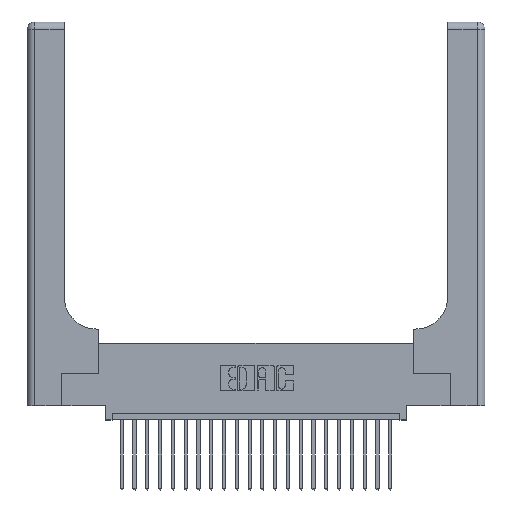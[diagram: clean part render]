
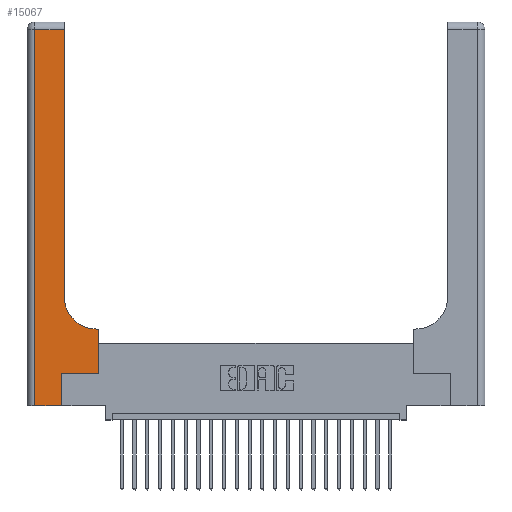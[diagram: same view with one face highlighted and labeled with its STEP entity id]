
A CAD part, top view. The second image highlights one B-rep face of the part: STEP entity #15067.
In plain terms, the highlighted planar face has unit normal (0, 0, 1).
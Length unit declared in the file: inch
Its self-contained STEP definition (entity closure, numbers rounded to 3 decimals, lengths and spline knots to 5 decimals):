
#415 = VECTOR ( 'NONE', #22402, 39.37008 ) ;
#859 = VECTOR ( 'NONE', #13262, 39.37008 ) ;
#1002 = LINE ( 'NONE', #6047, #415 ) ;
#1111 = PLANE ( 'NONE',  #16423 ) ;
#1129 = EDGE_CURVE ( 'NONE', #18419, #1137, #2459, .T. ) ;
#1137 = VERTEX_POINT ( 'NONE', #24298 ) ;
#1492 = CARTESIAN_POINT ( 'NONE',  ( 0., 0., 0.37 ) ) ;
#1927 = LINE ( 'NONE', #15598, #10284 ) ;
#2187 = CARTESIAN_POINT ( 'NONE',  ( 0.2915, 2.94, 0.37 ) ) ;
#2373 = ORIENTED_EDGE ( 'NONE', *, *, #10938, .T. ) ;
#2414 = CARTESIAN_POINT ( 'NONE',  ( 0.269, 0.25, 0.37 ) ) ;
#2459 = LINE ( 'NONE', #11232, #8430 ) ;
#2984 = DIRECTION ( 'NONE',  ( 1., 0., 0. ) ) ;
#3992 = CARTESIAN_POINT ( 'NONE',  ( 0.5415, 0.85, 0.37 ) ) ;
#4727 = CARTESIAN_POINT ( 'NONE',  ( 0.5585, 0.25, 0.37 ) ) ;
#5417 = VECTOR ( 'NONE', #24611, 39.37008 ) ;
#5508 = ORIENTED_EDGE ( 'NONE', *, *, #21727, .T. ) ;
#5813 = VERTEX_POINT ( 'NONE', #2414 ) ;
#6047 = CARTESIAN_POINT ( 'NONE',  ( 0.269, 0., 0.37 ) ) ;
#6265 = ORIENTED_EDGE ( 'NONE', *, *, #1129, .T. ) ;
#6415 = VECTOR ( 'NONE', #13257, 39.37008 ) ;
#6490 = ORIENTED_EDGE ( 'NONE', *, *, #20495, .T. ) ;
#6573 = VERTEX_POINT ( 'NONE', #10882 ) ;
#7051 = CARTESIAN_POINT ( 'NONE',  ( 0.06, 2.94, 0.37 ) ) ;
#7939 = VERTEX_POINT ( 'NONE', #13081 ) ;
#8109 = DIRECTION ( 'NONE',  ( -1., 0., 0. ) ) ;
#8239 = VECTOR ( 'NONE', #8879, 39.37008 ) ;
#8430 = VECTOR ( 'NONE', #18910, 39.37008 ) ;
#8801 = DIRECTION ( 'NONE',  ( -1., 0., 0. ) ) ;
#8806 = VERTEX_POINT ( 'NONE', #4727 ) ;
#8879 = DIRECTION ( 'NONE',  ( -1., 0., 0. ) ) ;
#10284 = VECTOR ( 'NONE', #8109, 39.37008 ) ;
#10451 = EDGE_CURVE ( 'NONE', #19938, #14213, #21950, .T. ) ;
#10579 = DIRECTION ( 'NONE',  ( 0., 0., -1. ) ) ;
#10651 = LINE ( 'NONE', #18865, #6415 ) ;
#10882 = CARTESIAN_POINT ( 'NONE',  ( 0.269, 0., 0.37 ) ) ;
#10901 = CARTESIAN_POINT ( 'NONE',  ( 0.2915, 0.85, 0.37 ) ) ;
#10938 = EDGE_CURVE ( 'NONE', #1137, #6573, #22531, .T. ) ;
#11232 = CARTESIAN_POINT ( 'NONE',  ( 0.06, 3., 0.37 ) ) ;
#11870 = FACE_OUTER_BOUND ( 'NONE', #13822, .T. ) ;
#11999 = CARTESIAN_POINT ( 'NONE',  ( 0.5415, 0.6, 0.37 ) ) ;
#12730 = ORIENTED_EDGE ( 'NONE', *, *, #15807, .T. ) ;
#13081 = CARTESIAN_POINT ( 'NONE',  ( 0.5585, 0.6, 0.37 ) ) ;
#13257 = DIRECTION ( 'NONE',  ( 0., 1., 0. ) ) ;
#13262 = DIRECTION ( 'NONE',  ( 1., 0., 0. ) ) ;
#13319 = LINE ( 'NONE', #23945, #8239 ) ;
#13822 = EDGE_LOOP ( 'NONE', ( #12730, #19896, #6265, #2373, #5508, #19318, #19345, #6490, #18004 ) ) ;
#14213 = VERTEX_POINT ( 'NONE', #10901 ) ;
#15067 = ADVANCED_FACE ( 'NONE', ( #11870 ), #1111, .F. ) ;
#15248 = EDGE_CURVE ( 'NONE', #8806, #7939, #23420, .T. ) ;
#15598 = CARTESIAN_POINT ( 'NONE',  ( 0., 2.94, 0.37 ) ) ;
#15807 = EDGE_CURVE ( 'NONE', #14213, #17592, #10651, .T. ) ;
#16172 = DIRECTION ( 'NONE',  ( 0., 1., 0. ) ) ;
#16423 = AXIS2_PLACEMENT_3D ( 'NONE', #24531, #20815, #8801 ) ;
#16464 = LINE ( 'NONE', #20610, #5417 ) ;
#17592 = VERTEX_POINT ( 'NONE', #2187 ) ;
#17596 = EDGE_CURVE ( 'NONE', #17592, #18419, #1927, .T. ) ;
#18004 = ORIENTED_EDGE ( 'NONE', *, *, #10451, .T. ) ;
#18374 = VECTOR ( 'NONE', #16172, 39.37008 ) ;
#18419 = VERTEX_POINT ( 'NONE', #7051 ) ;
#18865 = CARTESIAN_POINT ( 'NONE',  ( 0.2915, 3., 0.37 ) ) ;
#18910 = DIRECTION ( 'NONE',  ( 0., -1., 0. ) ) ;
#19318 = ORIENTED_EDGE ( 'NONE', *, *, #22276, .T. ) ;
#19345 = ORIENTED_EDGE ( 'NONE', *, *, #15248, .T. ) ;
#19896 = ORIENTED_EDGE ( 'NONE', *, *, #17596, .T. ) ;
#19938 = VERTEX_POINT ( 'NONE', #11999 ) ;
#20495 = EDGE_CURVE ( 'NONE', #7939, #19938, #13319, .T. ) ;
#20610 = CARTESIAN_POINT ( 'NONE',  ( 0.269, 0.25, 0.37 ) ) ;
#20815 = DIRECTION ( 'NONE',  ( 0., 0., -1. ) ) ;
#21727 = EDGE_CURVE ( 'NONE', #6573, #5813, #1002, .T. ) ;
#21832 = CARTESIAN_POINT ( 'NONE',  ( 0.5585, 0.25, 0.37 ) ) ;
#21950 = CIRCLE ( 'NONE', #24288, 0.25 ) ;
#22276 = EDGE_CURVE ( 'NONE', #5813, #8806, #16464, .T. ) ;
#22402 = DIRECTION ( 'NONE',  ( 0., 1., 0. ) ) ;
#22531 = LINE ( 'NONE', #1492, #859 ) ;
#23420 = LINE ( 'NONE', #21832, #18374 ) ;
#23945 = CARTESIAN_POINT ( 'NONE',  ( 0.2915, 0.6, 0.37 ) ) ;
#24288 = AXIS2_PLACEMENT_3D ( 'NONE', #3992, #10579, #2984 ) ;
#24298 = CARTESIAN_POINT ( 'NONE',  ( 0.06, 0., 0.37 ) ) ;
#24531 = CARTESIAN_POINT ( 'NONE',  ( 0., 3., 0.37 ) ) ;
#24611 = DIRECTION ( 'NONE',  ( 1., 0., 0. ) ) ;
